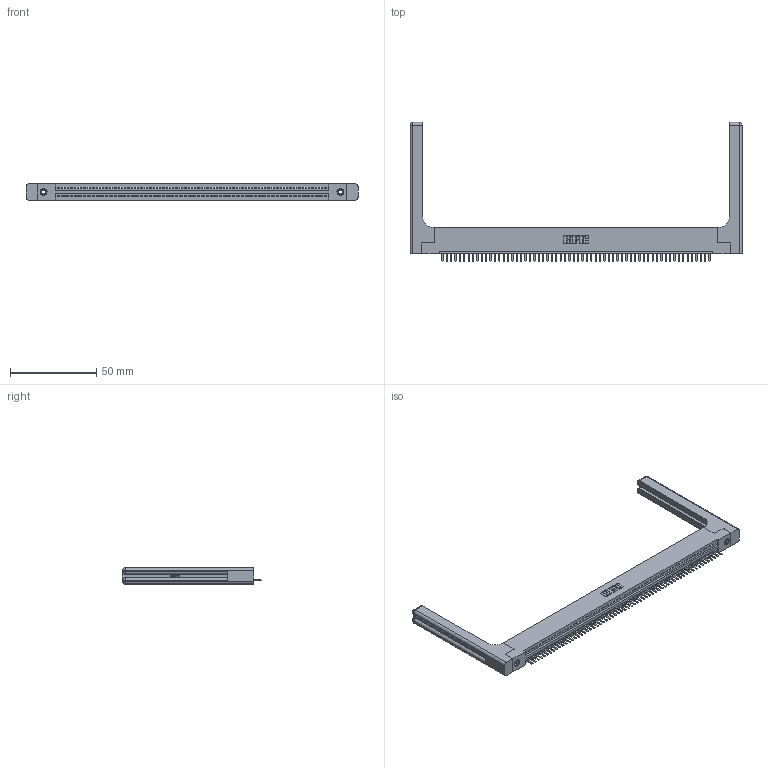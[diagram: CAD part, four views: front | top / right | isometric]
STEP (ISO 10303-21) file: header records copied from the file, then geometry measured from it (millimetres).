
FILE_DESCRIPTION (( 'STEP AP203' ), '1' );
FILE_NAME ('395-062-520-158.STEP', '2019-10-24T16:43:41', ( '' ), ( '' ), 'SwSTEP 2.0', 'SolidWorks 2016', '' );
FILE_SCHEMA (( 'CONFIG_CONTROL_DESIGN' ));
Length unit declared in the file: inch
Products named in the file (5): 345-250-001_345-250-001-102; 345-220-058_345-220-058; 345 Part_Flush Mounting Lugs - 0.156 Dia-TH; 395-062-520-158; 345-292-001_345-293-120
Assembly tree (67 placements, depth 2):
  395-062-520-158
    345 Part_Flush Mounting Lugs - 0.156 Dia-TH
    345-292-001_345-293-120  x62
    345-250-001_345-250-001-102  x2
    345-220-058_345-220-058  x2
Bounding box: 192.51 x 80.64 x 9.4 mm (x, y, z)
Volume: 26774.9 mm3; surface area: 29273.1 mm2
Topology: 67 solids, 67 shells, 4226 faces, 12415 edges, 8090 vertices
Faces by surface type: plane 2832, cylinder 1334, bspline 36, cone 12, sphere 8, torus 4
Entity records: 49266 total; most frequent: CARTESIAN_POINT 9515, ORIENTED_EDGE 8296, DIRECTION 7216, EDGE_CURVE 4148, LINE 3672, VECTOR 3672, VERTEX_POINT 2754, AXIS2_PLACEMENT_3D 1772
